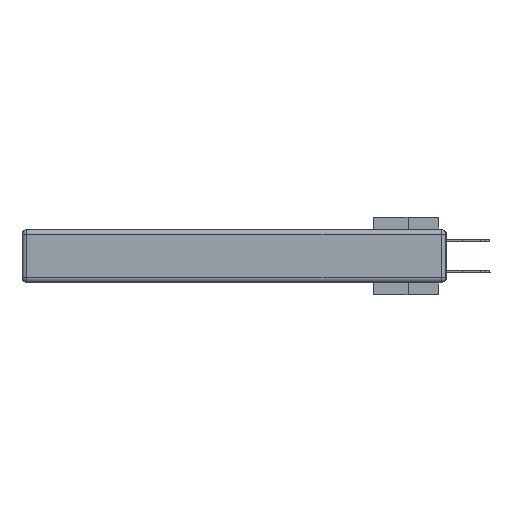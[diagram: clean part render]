
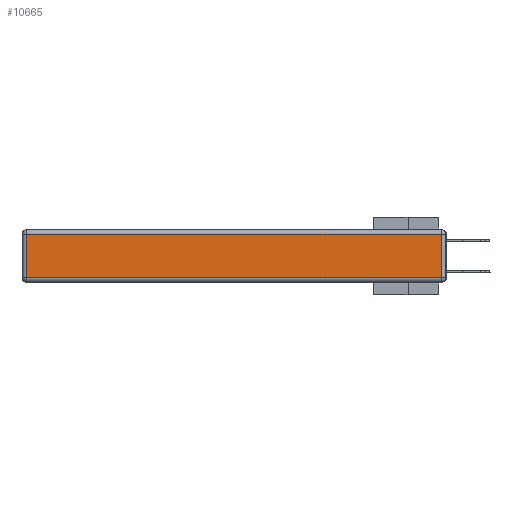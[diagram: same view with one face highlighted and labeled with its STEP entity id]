
A CAD part, left-side view. The second image highlights one B-rep face of the part: STEP entity #10665.
In plain terms, the highlighted planar face has unit normal (-1, 0, 0).
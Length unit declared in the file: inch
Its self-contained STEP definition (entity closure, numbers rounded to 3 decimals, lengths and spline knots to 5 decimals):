
#29 = DIRECTION ( 'NONE',  ( 0., 0., 1. ) ) ;
#600 = CARTESIAN_POINT ( 'NONE',  ( 0., 0., -0.343 ) ) ;
#1640 = VERTEX_POINT ( 'NONE', #36145 ) ;
#2821 = EDGE_CURVE ( 'NONE', #14660, #29413, #36576, .T. ) ;
#2915 = DIRECTION ( 'NONE',  ( 0., 0., -1. ) ) ;
#5972 = DIRECTION ( 'NONE',  ( 0., -1., 0. ) ) ;
#6582 = PLANE ( 'NONE',  #13793 ) ;
#6920 = LINE ( 'NONE', #23849, #19030 ) ;
#6976 = DIRECTION ( 'NONE',  ( -1., 0., 0. ) ) ;
#7179 = ORIENTED_EDGE ( 'NONE', *, *, #11458, .T. ) ;
#9055 = VERTEX_POINT ( 'NONE', #36625 ) ;
#10665 = ADVANCED_FACE ( 'NONE', ( #20542 ), #6582, .T. ) ;
#10955 = ORIENTED_EDGE ( 'NONE', *, *, #15541, .T. ) ;
#11458 = EDGE_CURVE ( 'NONE', #1640, #9055, #6920, .T. ) ;
#12364 = CARTESIAN_POINT ( 'NONE',  ( 0., 0.03, -0.343 ) ) ;
#13166 = LINE ( 'NONE', #12364, #32262 ) ;
#13793 = AXIS2_PLACEMENT_3D ( 'NONE', #600, #6976, #27433 ) ;
#14660 = VERTEX_POINT ( 'NONE', #23373 ) ;
#15074 = CARTESIAN_POINT ( 'NONE',  ( 0., 0., -0.313 ) ) ;
#15541 = EDGE_CURVE ( 'NONE', #29413, #1640, #13166, .T. ) ;
#16629 = VECTOR ( 'NONE', #2915, 39.37008 ) ;
#19030 = VECTOR ( 'NONE', #29870, 39.37008 ) ;
#19536 = EDGE_LOOP ( 'NONE', ( #36955, #10955, #7179, #20817 ) ) ;
#20542 = FACE_OUTER_BOUND ( 'NONE', #19536, .T. ) ;
#20817 = ORIENTED_EDGE ( 'NONE', *, *, #36801, .T. ) ;
#23373 = CARTESIAN_POINT ( 'NONE',  ( 0., 2.72, -0.313 ) ) ;
#23849 = CARTESIAN_POINT ( 'NONE',  ( 0., 2.75, -0.03 ) ) ;
#26907 = LINE ( 'NONE', #33189, #16629 ) ;
#27433 = DIRECTION ( 'NONE',  ( 0., 0., 1. ) ) ;
#29413 = VERTEX_POINT ( 'NONE', #32254 ) ;
#29870 = DIRECTION ( 'NONE',  ( 0., 1., 0. ) ) ;
#32254 = CARTESIAN_POINT ( 'NONE',  ( 0., 0.03, -0.313 ) ) ;
#32262 = VECTOR ( 'NONE', #29, 39.37008 ) ;
#33189 = CARTESIAN_POINT ( 'NONE',  ( 0., 2.72, -0.343 ) ) ;
#34203 = VECTOR ( 'NONE', #5972, 39.37008 ) ;
#36145 = CARTESIAN_POINT ( 'NONE',  ( 0., 0.03, -0.03 ) ) ;
#36576 = LINE ( 'NONE', #15074, #34203 ) ;
#36625 = CARTESIAN_POINT ( 'NONE',  ( 0., 2.72, -0.03 ) ) ;
#36801 = EDGE_CURVE ( 'NONE', #9055, #14660, #26907, .T. ) ;
#36955 = ORIENTED_EDGE ( 'NONE', *, *, #2821, .T. ) ;
